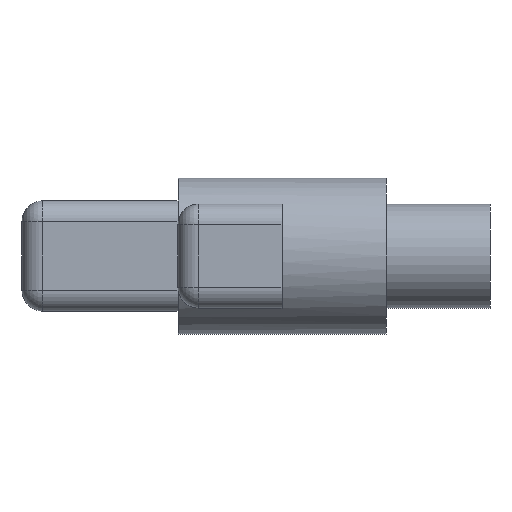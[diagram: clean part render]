
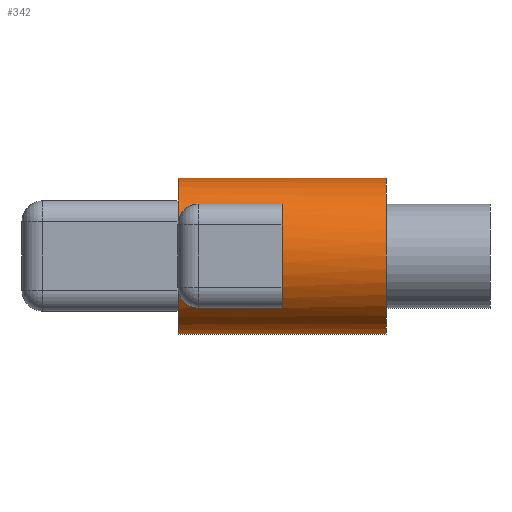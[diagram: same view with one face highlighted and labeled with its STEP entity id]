
A CAD part, left-side view. The second image highlights one B-rep face of the part: STEP entity #342.
In plain terms, the highlighted cylindrical face has radius 7.5 mm (diameter 15 mm), a partial arc.
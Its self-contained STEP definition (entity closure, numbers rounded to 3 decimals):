
#11 = DIRECTION ( 'NONE',  ( 0., 0., -1. ) ) ;
#15 = CARTESIAN_POINT ( 'NONE',  ( -6.874, 20., 3. ) ) ;
#24 = CARTESIAN_POINT ( 'NONE',  ( -5.604, 18.288, 4.984 ) ) ;
#39 = CARTESIAN_POINT ( 'NONE',  ( -6.874, 20., 3. ) ) ;
#73 = VERTEX_POINT ( 'NONE', #830 ) ;
#84 = DIRECTION ( 'NONE',  ( 0., -1., 0. ) ) ;
#88 = CARTESIAN_POINT ( 'NONE',  ( -5.59, 18., -5. ) ) ;
#90 = DIRECTION ( 'NONE',  ( 0., 0., 1. ) ) ;
#91 = DIRECTION ( 'NONE',  ( 0., 1., 0. ) ) ;
#94 = DIRECTION ( 'NONE',  ( 0., 1., 0. ) ) ;
#98 = CARTESIAN_POINT ( 'NONE',  ( 0., 20., 0. ) ) ;
#122 = CARTESIAN_POINT ( 'NONE',  ( -5.957, 19.275, 4.562 ) ) ;
#147 = CARTESIAN_POINT ( 'NONE',  ( -5.657, 18.564, 4.924 ) ) ;
#189 = CARTESIAN_POINT ( 'NONE',  ( -6.629, 19.938, -3.51 ) ) ;
#192 = LINE ( 'NONE', #394, #198 ) ;
#198 = VECTOR ( 'NONE', #1019, 1000. ) ;
#205 = CARTESIAN_POINT ( 'NONE',  ( 0., 0., 0. ) ) ;
#211 = CARTESIAN_POINT ( 'NONE',  ( 0., 10., 0. ) ) ;
#229 = VERTEX_POINT ( 'NONE', #688 ) ;
#307 = CARTESIAN_POINT ( 'NONE',  ( -6.428, 19.807, -3.866 ) ) ;
#315 = CARTESIAN_POINT ( 'NONE',  ( 0., 20., 0. ) ) ;
#335 = CARTESIAN_POINT ( 'NONE',  ( -5.59, 18., 5. ) ) ;
#336 = DIRECTION ( 'NONE',  ( 0., 0., -1. ) ) ;
#342 = ADVANCED_FACE ( 'NONE', ( #752 ), #747, .T. ) ;
#344 = VECTOR ( 'NONE', #84, 1000. ) ;
#346 = VECTOR ( 'NONE', #91, 1000. ) ;
#352 = DIRECTION ( 'NONE',  ( 0., -1., 0. ) ) ;
#359 = LINE ( 'NONE', #1157, #346 ) ;
#365 = LINE ( 'NONE', #884, #344 ) ;
#394 = CARTESIAN_POINT ( 'NONE',  ( -5.59, 20., 5. ) ) ;
#397 = CIRCLE ( 'NONE', #1262, 7.5 ) ;
#415 = ORIENTED_EDGE ( 'NONE', *, *, #986, .T. ) ;
#429 = CARTESIAN_POINT ( 'NONE',  ( -6.224, 19.614, -4.187 ) ) ;
#430 = EDGE_CURVE ( 'NONE', #700, #1212, #681, .T. ) ;
#434 = CARTESIAN_POINT ( 'NONE',  ( -5.604, 18.285, -4.985 ) ) ;
#438 = B_SPLINE_CURVE_WITH_KNOTS ( 'NONE', 3,
 ( #88, #556, #434, #775, #1381, #886, #1261, #550, #664, #1151, #429, #1042, #307, #968, #189, #881, #774, #1375 ),
 .UNSPECIFIED., .F., .F.,
 ( 4, 2, 2, 2, 2, 2, 2, 2, 4 ),
 ( 0., 0., 0.001, 0.001, 0.002, 0.002, 0.003, 0.003, 0.003 ),
 .UNSPECIFIED. ) ;
#464 = VERTEX_POINT ( 'NONE', #39 ) ;
#485 = CARTESIAN_POINT ( 'NONE',  ( -6.632, 19.949, 3.514 ) ) ;
#489 = CARTESIAN_POINT ( 'NONE',  ( -5.59, 10., 5. ) ) ;
#497 = VECTOR ( 'NONE', #611, 1000. ) ;
#498 = LINE ( 'NONE', #831, #497 ) ;
#508 = EDGE_CURVE ( 'NONE', #464, #825, #1210, .T. ) ;
#550 = CARTESIAN_POINT ( 'NONE',  ( -5.96, 19.266, -4.554 ) ) ;
#556 = CARTESIAN_POINT ( 'NONE',  ( -5.59, 18.144, -5. ) ) ;
#560 = DIRECTION ( 'NONE',  ( 0., 0., 1. ) ) ;
#561 = EDGE_CURVE ( 'NONE', #903, #1212, #438, .T. ) ;
#567 = CIRCLE ( 'NONE', #1183, 7.5 ) ;
#607 = CARTESIAN_POINT ( 'NONE',  ( 0., 20., -7.5 ) ) ;
#611 = DIRECTION ( 'NONE',  ( 0., -1., 0. ) ) ;
#628 = CARTESIAN_POINT ( 'NONE',  ( -5.695, 18.694, 4.881 ) ) ;
#645 = EDGE_CURVE ( 'NONE', #1169, #1071, #567, .T. ) ;
#664 = CARTESIAN_POINT ( 'NONE',  ( -6.023, 19.362, -4.47 ) ) ;
#672 = CARTESIAN_POINT ( 'NONE',  ( 0., 20., 0. ) ) ;
#681 = CIRCLE ( 'NONE', #1003, 7.5 ) ;
#688 = CARTESIAN_POINT ( 'NONE',  ( -5.59, 18., 5. ) ) ;
#700 = VERTEX_POINT ( 'NONE', #607 ) ;
#721 = EDGE_CURVE ( 'NONE', #825, #1250, #498, .T. ) ;
#746 = CARTESIAN_POINT ( 'NONE',  ( 0., 20., 7.5 ) ) ;
#747 = CYLINDRICAL_SURFACE ( 'NONE', #1251, 7.5 ) ;
#752 = FACE_OUTER_BOUND ( 'NONE', #1383, .T. ) ;
#774 = CARTESIAN_POINT ( 'NONE',  ( -6.816, 20., -3.132 ) ) ;
#775 = CARTESIAN_POINT ( 'NONE',  ( -5.656, 18.559, -4.925 ) ) ;
#825 = VERTEX_POINT ( 'NONE', #746 ) ;
#826 = CARTESIAN_POINT ( 'NONE',  ( -6.759, 20., 3.264 ) ) ;
#830 = CARTESIAN_POINT ( 'NONE',  ( 0., 0., -7.5 ) ) ;
#831 = CARTESIAN_POINT ( 'NONE',  ( 0., 20., 7.5 ) ) ;
#844 = CARTESIAN_POINT ( 'NONE',  ( -6.222, 19.625, 4.194 ) ) ;
#881 = CARTESIAN_POINT ( 'NONE',  ( -6.756, 19.987, -3.26 ) ) ;
#884 = CARTESIAN_POINT ( 'NONE',  ( 0., 20., -7.5 ) ) ;
#886 = CARTESIAN_POINT ( 'NONE',  ( -5.787, 18.938, -4.771 ) ) ;
#891 = DIRECTION ( 'NONE',  ( 0., 1., 0. ) ) ;
#903 = VERTEX_POINT ( 'NONE', #1028 ) ;
#920 = AXIS2_PLACEMENT_3D ( 'NONE', #672, #1275, #560 ) ;
#929 = EDGE_CURVE ( 'NONE', #73, #1250, #397, .T. ) ;
#950 = B_SPLINE_CURVE_WITH_KNOTS ( 'NONE', 3,
 ( #15, #826, #485, #1092, #844, #122, #1342, #628, #147, #24, #1062, #335 ),
 .UNSPECIFIED., .F., .F.,
 ( 4, 2, 2, 2, 2, 4 ),
 ( 0., 0.001, 0.002, 0.003, 0.003, 0.003 ),
 .UNSPECIFIED. ) ;
#968 = CARTESIAN_POINT ( 'NONE',  ( -6.563, 19.901, -3.633 ) ) ;
#975 = DIRECTION ( 'NONE',  ( 0., 0., 1. ) ) ;
#981 = EDGE_CURVE ( 'NONE', #1071, #903, #359, .T. ) ;
#985 = CARTESIAN_POINT ( 'NONE',  ( -6.874, 20., -3. ) ) ;
#986 = EDGE_CURVE ( 'NONE', #700, #73, #365, .T. ) ;
#993 = DIRECTION ( 'NONE',  ( 0., -1., 0. ) ) ;
#1003 = AXIS2_PLACEMENT_3D ( 'NONE', #98, #94, #90 ) ;
#1019 = DIRECTION ( 'NONE',  ( 0., -1., 0. ) ) ;
#1028 = CARTESIAN_POINT ( 'NONE',  ( -5.59, 18., -5. ) ) ;
#1033 = ORIENTED_EDGE ( 'NONE', *, *, #981, .T. ) ;
#1042 = CARTESIAN_POINT ( 'NONE',  ( -6.36, 19.75, -3.977 ) ) ;
#1062 = CARTESIAN_POINT ( 'NONE',  ( -5.59, 18.145, 5. ) ) ;
#1071 = VERTEX_POINT ( 'NONE', #1364 ) ;
#1085 = ORIENTED_EDGE ( 'NONE', *, *, #1172, .T. ) ;
#1092 = CARTESIAN_POINT ( 'NONE',  ( -6.361, 19.76, 3.983 ) ) ;
#1122 = ORIENTED_EDGE ( 'NONE', *, *, #721, .F. ) ;
#1151 = CARTESIAN_POINT ( 'NONE',  ( -6.155, 19.536, -4.287 ) ) ;
#1157 = CARTESIAN_POINT ( 'NONE',  ( -5.59, 20., -5. ) ) ;
#1169 = VERTEX_POINT ( 'NONE', #489 ) ;
#1172 = EDGE_CURVE ( 'NONE', #464, #229, #950, .T. ) ;
#1183 = AXIS2_PLACEMENT_3D ( 'NONE', #211, #993, #11 ) ;
#1210 = CIRCLE ( 'NONE', #920, 7.5 ) ;
#1212 = VERTEX_POINT ( 'NONE', #985 ) ;
#1250 = VERTEX_POINT ( 'NONE', #1335 ) ;
#1251 = AXIS2_PLACEMENT_3D ( 'NONE', #315, #352, #336 ) ;
#1261 = CARTESIAN_POINT ( 'NONE',  ( -5.842, 19.055, -4.704 ) ) ;
#1262 = AXIS2_PLACEMENT_3D ( 'NONE', #205, #891, #975 ) ;
#1275 = DIRECTION ( 'NONE',  ( 0., 1., 0. ) ) ;
#1284 = ORIENTED_EDGE ( 'NONE', *, *, #561, .T. ) ;
#1307 = ORIENTED_EDGE ( 'NONE', *, *, #508, .F. ) ;
#1311 = ORIENTED_EDGE ( 'NONE', *, *, #1326, .T. ) ;
#1323 = ORIENTED_EDGE ( 'NONE', *, *, #645, .T. ) ;
#1326 = EDGE_CURVE ( 'NONE', #229, #1169, #192, .T. ) ;
#1335 = CARTESIAN_POINT ( 'NONE',  ( 0., 0., 7.5 ) ) ;
#1342 = CARTESIAN_POINT ( 'NONE',  ( -5.836, 19.067, 4.714 ) ) ;
#1356 = ORIENTED_EDGE ( 'NONE', *, *, #430, .F. ) ;
#1364 = CARTESIAN_POINT ( 'NONE',  ( -5.59, 10., -5. ) ) ;
#1375 = CARTESIAN_POINT ( 'NONE',  ( -6.874, 20., -3. ) ) ;
#1381 = CARTESIAN_POINT ( 'NONE',  ( -5.695, 18.692, -4.881 ) ) ;
#1383 = EDGE_LOOP ( 'NONE', ( #1122, #1307, #1085, #1311, #1323, #1033, #1284, #1356, #415, #1385 ) ) ;
#1385 = ORIENTED_EDGE ( 'NONE', *, *, #929, .T. ) ;
